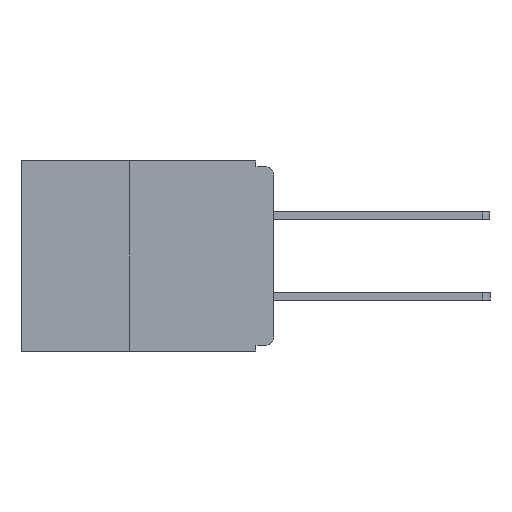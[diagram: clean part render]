
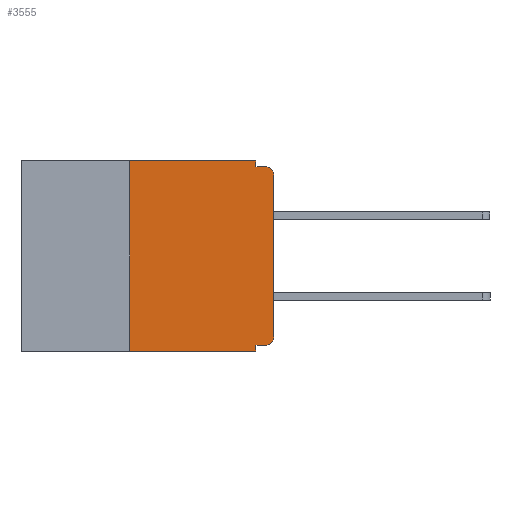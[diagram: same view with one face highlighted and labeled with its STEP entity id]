
A CAD part, left-side view. The second image highlights one B-rep face of the part: STEP entity #3555.
In plain terms, the highlighted planar face has unit normal (-1, 0, 0).
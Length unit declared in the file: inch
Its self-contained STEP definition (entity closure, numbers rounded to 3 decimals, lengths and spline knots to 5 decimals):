
#8 = CARTESIAN_POINT ( 'NONE',  ( 0., 0.25, -0.33 ) ) ;
#68 = DIRECTION ( 'NONE',  ( 0., 0., -1. ) ) ;
#1072 = DIRECTION ( 'NONE',  ( 0., 0., -1. ) ) ;
#1230 = VECTOR ( 'NONE', #12893, 39.37008 ) ;
#1588 = DIRECTION ( 'NONE',  ( 1., 0., 0. ) ) ;
#1669 = LINE ( 'NONE', #9330, #15616 ) ;
#2244 = FACE_OUTER_BOUND ( 'NONE', #11831, .T. ) ;
#2544 = VECTOR ( 'NONE', #17436, 39.37008 ) ;
#2699 = PLANE ( 'NONE',  #24605 ) ;
#2751 = EDGE_CURVE ( 'NONE', #3055, #19063, #24798, .T. ) ;
#3055 = VERTEX_POINT ( 'NONE', #15671 ) ;
#3555 = ADVANCED_FACE ( 'NONE', ( #2244 ), #2699, .F. ) ;
#3594 = CARTESIAN_POINT ( 'NONE',  ( 0., 0.031, -0.32 ) ) ;
#3735 = EDGE_CURVE ( 'NONE', #24285, #3943, #18280, .T. ) ;
#3943 = VERTEX_POINT ( 'NONE', #8872 ) ;
#4154 = VERTEX_POINT ( 'NONE', #8 ) ;
#4348 = VECTOR ( 'NONE', #18454, 39.37008 ) ;
#4413 = EDGE_CURVE ( 'NONE', #14388, #13420, #22784, .T. ) ;
#4632 = CARTESIAN_POINT ( 'NONE',  ( 0., 0.437, 0. ) ) ;
#4881 = CARTESIAN_POINT ( 'NONE',  ( 0., 0., 0. ) ) ;
#4958 = DIRECTION ( 'NONE',  ( 0., 0., -1. ) ) ;
#4994 = ORIENTED_EDGE ( 'NONE', *, *, #12376, .T. ) ;
#5420 = AXIS2_PLACEMENT_3D ( 'NONE', #5549, #19335, #7557 ) ;
#5549 = CARTESIAN_POINT ( 'NONE',  ( 0., 0.015, -0.025 ) ) ;
#5718 = EDGE_CURVE ( 'NONE', #4154, #13420, #14276, .T. ) ;
#5769 = ORIENTED_EDGE ( 'NONE', *, *, #12571, .T. ) ;
#6059 = CARTESIAN_POINT ( 'NONE',  ( 0., 0., -0.025 ) ) ;
#6215 = ORIENTED_EDGE ( 'NONE', *, *, #3735, .F. ) ;
#6896 = ORIENTED_EDGE ( 'NONE', *, *, #9748, .F. ) ;
#7056 = EDGE_CURVE ( 'NONE', #4154, #7421, #18131, .T. ) ;
#7421 = VERTEX_POINT ( 'NONE', #7994 ) ;
#7557 = DIRECTION ( 'NONE',  ( 0., 0., -1. ) ) ;
#7994 = CARTESIAN_POINT ( 'NONE',  ( 0., 0.25, 0. ) ) ;
#8416 = ORIENTED_EDGE ( 'NONE', *, *, #9013, .F. ) ;
#8576 = EDGE_CURVE ( 'NONE', #3055, #14388, #20187, .T. ) ;
#8701 = CIRCLE ( 'NONE', #5420, 0.015 ) ;
#8872 = CARTESIAN_POINT ( 'NONE',  ( 0., 0.015, -0.01 ) ) ;
#8994 = DIRECTION ( 'NONE',  ( 0., 0., 1. ) ) ;
#9013 = EDGE_CURVE ( 'NONE', #7421, #21468, #1669, .T. ) ;
#9330 = CARTESIAN_POINT ( 'NONE',  ( 0., 0.437, 0. ) ) ;
#9748 = EDGE_CURVE ( 'NONE', #21468, #24285, #22247, .T. ) ;
#9927 = AXIS2_PLACEMENT_3D ( 'NONE', #11352, #11514, #68 ) ;
#10031 = ORIENTED_EDGE ( 'NONE', *, *, #7056, .F. ) ;
#10139 = ORIENTED_EDGE ( 'NONE', *, *, #5718, .T. ) ;
#10419 = VECTOR ( 'NONE', #11759, 39.37008 ) ;
#10822 = ORIENTED_EDGE ( 'NONE', *, *, #4413, .F. ) ;
#11239 = ORIENTED_EDGE ( 'NONE', *, *, #8576, .F. ) ;
#11352 = CARTESIAN_POINT ( 'NONE',  ( 0., 0.015, -0.305 ) ) ;
#11514 = DIRECTION ( 'NONE',  ( -1., 0., 0. ) ) ;
#11759 = DIRECTION ( 'NONE',  ( 0., 1., 0. ) ) ;
#11831 = EDGE_LOOP ( 'NONE', ( #4994, #5769, #6215, #6896, #8416, #10031, #10139, #10822, #11239, #12228 ) ) ;
#12201 = CARTESIAN_POINT ( 'NONE',  ( 0., 0.031, 0. ) ) ;
#12228 = ORIENTED_EDGE ( 'NONE', *, *, #2751, .T. ) ;
#12376 = EDGE_CURVE ( 'NONE', #19063, #12729, #17591, .T. ) ;
#12571 = EDGE_CURVE ( 'NONE', #12729, #3943, #8701, .T. ) ;
#12729 = VERTEX_POINT ( 'NONE', #6059 ) ;
#12881 = CARTESIAN_POINT ( 'NONE',  ( 0., 0.031, 0. ) ) ;
#12893 = DIRECTION ( 'NONE',  ( 0., 0., 1. ) ) ;
#13420 = VERTEX_POINT ( 'NONE', #19883 ) ;
#13727 = VECTOR ( 'NONE', #19683, 39.37008 ) ;
#14276 = LINE ( 'NONE', #18591, #4348 ) ;
#14388 = VERTEX_POINT ( 'NONE', #3594 ) ;
#14601 = CARTESIAN_POINT ( 'NONE',  ( 0., 0.031, -0.01 ) ) ;
#15616 = VECTOR ( 'NONE', #22929, 39.37008 ) ;
#15671 = CARTESIAN_POINT ( 'NONE',  ( 0., 0.015, -0.32 ) ) ;
#16329 = CARTESIAN_POINT ( 'NONE',  ( 0., 0., -0.305 ) ) ;
#16613 = CARTESIAN_POINT ( 'NONE',  ( 0., 0., -0.01 ) ) ;
#17436 = DIRECTION ( 'NONE',  ( 0., -1., 0. ) ) ;
#17591 = LINE ( 'NONE', #4881, #1230 ) ;
#18131 = LINE ( 'NONE', #24555, #24478 ) ;
#18280 = LINE ( 'NONE', #16613, #2544 ) ;
#18454 = DIRECTION ( 'NONE',  ( 0., -1., 0. ) ) ;
#18591 = CARTESIAN_POINT ( 'NONE',  ( 0., 0.437, -0.33 ) ) ;
#19063 = VERTEX_POINT ( 'NONE', #16329 ) ;
#19335 = DIRECTION ( 'NONE',  ( -1., 0., 0. ) ) ;
#19683 = DIRECTION ( 'NONE',  ( 0., 0., -1. ) ) ;
#19703 = CARTESIAN_POINT ( 'NONE',  ( 0., 0.031, -0.33 ) ) ;
#19883 = CARTESIAN_POINT ( 'NONE',  ( 0., 0.031, -0.33 ) ) ;
#20187 = LINE ( 'NONE', #21606, #10419 ) ;
#21468 = VERTEX_POINT ( 'NONE', #12201 ) ;
#21606 = CARTESIAN_POINT ( 'NONE',  ( 0., 0., -0.32 ) ) ;
#21652 = VECTOR ( 'NONE', #4958, 39.37008 ) ;
#22247 = LINE ( 'NONE', #12881, #21652 ) ;
#22784 = LINE ( 'NONE', #19703, #13727 ) ;
#22929 = DIRECTION ( 'NONE',  ( 0., -1., 0. ) ) ;
#24285 = VERTEX_POINT ( 'NONE', #14601 ) ;
#24478 = VECTOR ( 'NONE', #8994, 39.37008 ) ;
#24555 = CARTESIAN_POINT ( 'NONE',  ( 0., 0.25, -0.33 ) ) ;
#24605 = AXIS2_PLACEMENT_3D ( 'NONE', #4632, #1588, #1072 ) ;
#24798 = CIRCLE ( 'NONE', #9927, 0.015 ) ;
